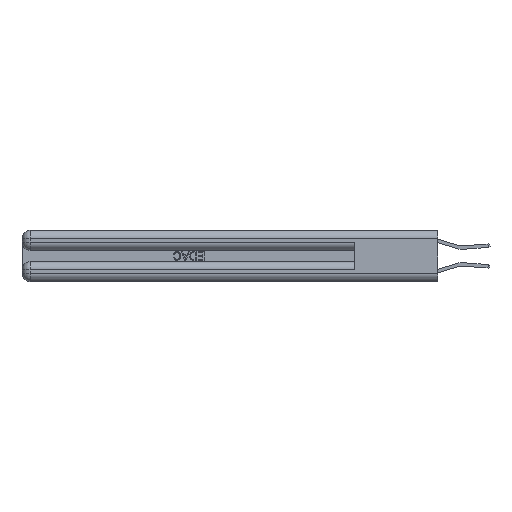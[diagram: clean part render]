
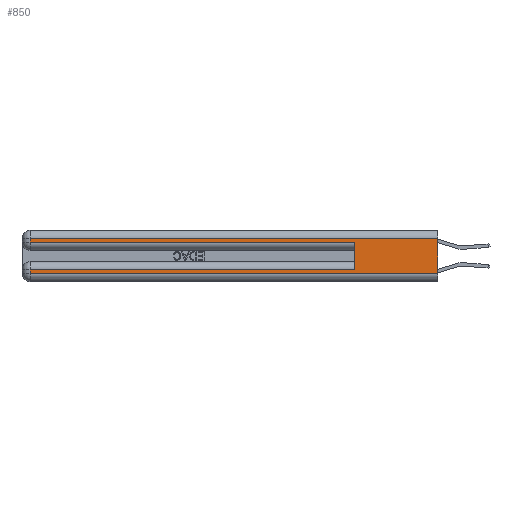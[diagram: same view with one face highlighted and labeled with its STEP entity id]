
A CAD part, left-side view. The second image highlights one B-rep face of the part: STEP entity #850.
In plain terms, the highlighted planar face has unit normal (-1, 0, 0).
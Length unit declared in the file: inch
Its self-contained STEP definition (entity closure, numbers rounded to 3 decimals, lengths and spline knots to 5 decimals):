
#113 = EDGE_CURVE ( 'NONE', #26116, #13017, #4060, .T. ) ;
#431 = CARTESIAN_POINT ( 'NONE',  ( 0., 2.94, 0.085 ) ) ;
#466 = EDGE_CURVE ( 'NONE', #8871, #12170, #27967, .T. ) ;
#688 = VECTOR ( 'NONE', #28677, 39.37008 ) ;
#850 = ADVANCED_FACE ( 'NONE', ( #16901 ), #27894, .F. ) ;
#1786 = DIRECTION ( 'NONE',  ( 0., 0., -1. ) ) ;
#1893 = CARTESIAN_POINT ( 'NONE',  ( 0., 2.94, 0.31 ) ) ;
#2045 = DIRECTION ( 'NONE',  ( 0., -1., 0. ) ) ;
#2169 = EDGE_CURVE ( 'NONE', #28812, #6993, #4629, .T. ) ;
#2185 = CARTESIAN_POINT ( 'NONE',  ( 0., 0., 0.31 ) ) ;
#3107 = ORIENTED_EDGE ( 'NONE', *, *, #3309, .F. ) ;
#3309 = EDGE_CURVE ( 'NONE', #13539, #6993, #13873, .T. ) ;
#3329 = EDGE_LOOP ( 'NONE', ( #10430, #8747, #23143, #25960, #3107, #14896, #25089, #8027 ) ) ;
#3413 = AXIS2_PLACEMENT_3D ( 'NONE', #9931, #18868, #12227 ) ;
#3892 = LINE ( 'NONE', #23937, #25677 ) ;
#4060 = LINE ( 'NONE', #26383, #27644 ) ;
#4629 = LINE ( 'NONE', #8976, #11799 ) ;
#5471 = EDGE_CURVE ( 'NONE', #25648, #8871, #23963, .T. ) ;
#5845 = CARTESIAN_POINT ( 'NONE',  ( 0., 2.94, 0.285 ) ) ;
#6982 = EDGE_CURVE ( 'NONE', #26116, #12170, #9575, .T. ) ;
#6993 = VERTEX_POINT ( 'NONE', #17982 ) ;
#7261 = CARTESIAN_POINT ( 'NONE',  ( 0., 0., 0.37 ) ) ;
#7321 = VECTOR ( 'NONE', #22252, 39.37008 ) ;
#8027 = ORIENTED_EDGE ( 'NONE', *, *, #466, .T. ) ;
#8747 = ORIENTED_EDGE ( 'NONE', *, *, #113, .T. ) ;
#8871 = VERTEX_POINT ( 'NONE', #18123 ) ;
#8976 = CARTESIAN_POINT ( 'NONE',  ( 0., 0., 0.285 ) ) ;
#9575 = LINE ( 'NONE', #7261, #20327 ) ;
#9931 = CARTESIAN_POINT ( 'NONE',  ( 0., 0., 0.37 ) ) ;
#10430 = ORIENTED_EDGE ( 'NONE', *, *, #6982, .F. ) ;
#10975 = CARTESIAN_POINT ( 'NONE',  ( 0., 0.6, 0.145 ) ) ;
#11799 = VECTOR ( 'NONE', #24776, 39.37008 ) ;
#12170 = VERTEX_POINT ( 'NONE', #15016 ) ;
#12227 = DIRECTION ( 'NONE',  ( 0., 0., -1. ) ) ;
#12582 = CARTESIAN_POINT ( 'NONE',  ( 0., 0.6, 0.085 ) ) ;
#12720 = DIRECTION ( 'NONE',  ( 0., 1., 0. ) ) ;
#13017 = VERTEX_POINT ( 'NONE', #1893 ) ;
#13161 = DIRECTION ( 'NONE',  ( 0., 0., 1. ) ) ;
#13175 = VECTOR ( 'NONE', #13161, 39.37008 ) ;
#13539 = VERTEX_POINT ( 'NONE', #12582 ) ;
#13873 = LINE ( 'NONE', #10975, #13175 ) ;
#14745 = VECTOR ( 'NONE', #2045, 39.37008 ) ;
#14896 = ORIENTED_EDGE ( 'NONE', *, *, #22322, .T. ) ;
#15016 = CARTESIAN_POINT ( 'NONE',  ( 0., 0., 0.06 ) ) ;
#15762 = CARTESIAN_POINT ( 'NONE',  ( 0., 2.94, 0.37 ) ) ;
#15918 = CARTESIAN_POINT ( 'NONE',  ( 0., 0., 0.06 ) ) ;
#16901 = FACE_OUTER_BOUND ( 'NONE', #3329, .T. ) ;
#17982 = CARTESIAN_POINT ( 'NONE',  ( 0., 0.6, 0.285 ) ) ;
#18086 = LINE ( 'NONE', #15762, #7321 ) ;
#18123 = CARTESIAN_POINT ( 'NONE',  ( 0., 2.94, 0.06 ) ) ;
#18868 = DIRECTION ( 'NONE',  ( 1., 0., 0. ) ) ;
#20327 = VECTOR ( 'NONE', #1786, 39.37008 ) ;
#22252 = DIRECTION ( 'NONE',  ( 0., 0., -1. ) ) ;
#22322 = EDGE_CURVE ( 'NONE', #13539, #25648, #3892, .T. ) ;
#23143 = ORIENTED_EDGE ( 'NONE', *, *, #27265, .T. ) ;
#23937 = CARTESIAN_POINT ( 'NONE',  ( 0., 0., 0.085 ) ) ;
#23963 = LINE ( 'NONE', #28882, #688 ) ;
#24234 = DIRECTION ( 'NONE',  ( 0., 1., 0. ) ) ;
#24776 = DIRECTION ( 'NONE',  ( 0., -1., 0. ) ) ;
#25089 = ORIENTED_EDGE ( 'NONE', *, *, #5471, .T. ) ;
#25648 = VERTEX_POINT ( 'NONE', #431 ) ;
#25677 = VECTOR ( 'NONE', #24234, 39.37008 ) ;
#25960 = ORIENTED_EDGE ( 'NONE', *, *, #2169, .T. ) ;
#26116 = VERTEX_POINT ( 'NONE', #2185 ) ;
#26383 = CARTESIAN_POINT ( 'NONE',  ( 0., 0., 0.31 ) ) ;
#27265 = EDGE_CURVE ( 'NONE', #13017, #28812, #18086, .T. ) ;
#27644 = VECTOR ( 'NONE', #12720, 39.37008 ) ;
#27894 = PLANE ( 'NONE',  #3413 ) ;
#27967 = LINE ( 'NONE', #15918, #14745 ) ;
#28677 = DIRECTION ( 'NONE',  ( 0., 0., -1. ) ) ;
#28812 = VERTEX_POINT ( 'NONE', #5845 ) ;
#28882 = CARTESIAN_POINT ( 'NONE',  ( 0., 2.94, 0.37 ) ) ;
